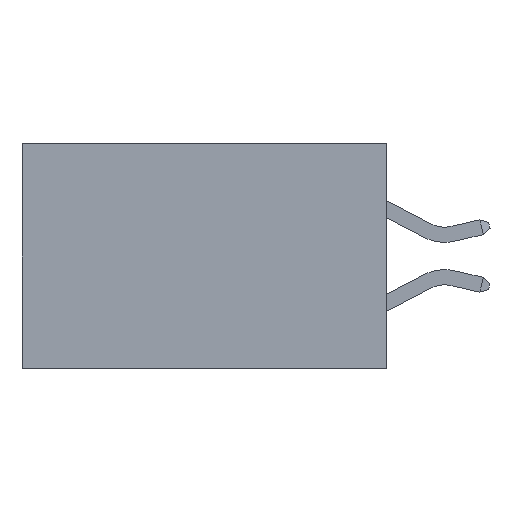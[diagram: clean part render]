
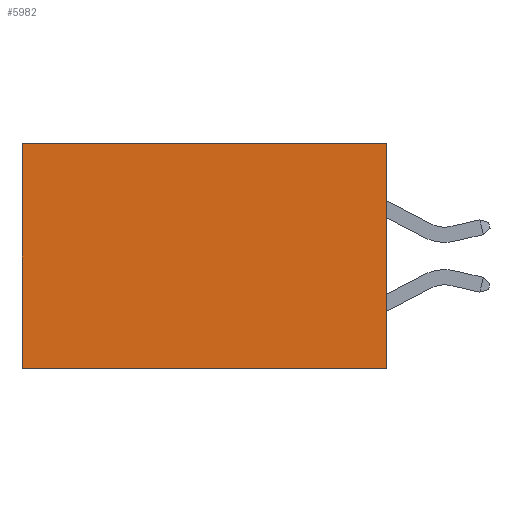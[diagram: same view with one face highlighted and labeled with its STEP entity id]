
A CAD part, left-side view. The second image highlights one B-rep face of the part: STEP entity #5982.
In plain terms, the highlighted planar face has unit normal (-1, 0, 0).
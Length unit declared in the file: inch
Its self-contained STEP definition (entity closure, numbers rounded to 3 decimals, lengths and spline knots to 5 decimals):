
#1106 = EDGE_CURVE ( 'NONE', #20716, #8782, #17215, .T. ) ;
#1130 = ORIENTED_EDGE ( 'NONE', *, *, #15446, .F. ) ;
#2892 = VERTEX_POINT ( 'NONE', #3396 ) ;
#3396 = CARTESIAN_POINT ( 'NONE',  ( 0.2615, 0., -0.37 ) ) ;
#3683 = DIRECTION ( 'NONE',  ( 0., 0., -1. ) ) ;
#3804 = PLANE ( 'NONE',  #22544 ) ;
#4416 = EDGE_CURVE ( 'NONE', #2892, #8782, #11045, .T. ) ;
#4442 = DIRECTION ( 'NONE',  ( 0., 0., -1. ) ) ;
#5888 = DIRECTION ( 'NONE',  ( 0., 0., -1. ) ) ;
#5982 = ADVANCED_FACE ( 'NONE', ( #23547 ), #3804, .F. ) ;
#6542 = VECTOR ( 'NONE', #4442, 39.37008 ) ;
#6616 = LINE ( 'NONE', #6861, #24204 ) ;
#6861 = CARTESIAN_POINT ( 'NONE',  ( 0.2615, 0., 0. ) ) ;
#7261 = VECTOR ( 'NONE', #9505, 39.37008 ) ;
#8311 = CARTESIAN_POINT ( 'NONE',  ( 0.2615, 0.6, 0. ) ) ;
#8782 = VERTEX_POINT ( 'NONE', #24409 ) ;
#9505 = DIRECTION ( 'NONE',  ( 0., 1., 0. ) ) ;
#10264 = CARTESIAN_POINT ( 'NONE',  ( 0.2615, 0., -0.37 ) ) ;
#11045 = LINE ( 'NONE', #14894, #7261 ) ;
#11678 = CARTESIAN_POINT ( 'NONE',  ( 0.2615, 0., -0.37 ) ) ;
#11791 = CARTESIAN_POINT ( 'NONE',  ( 0.2615, 0.6, -0.37 ) ) ;
#12699 = LINE ( 'NONE', #10264, #6542 ) ;
#13491 = ORIENTED_EDGE ( 'NONE', *, *, #18817, .T. ) ;
#14714 = DIRECTION ( 'NONE',  ( 0., 1., 0. ) ) ;
#14894 = CARTESIAN_POINT ( 'NONE',  ( 0.2615, 0., -0.37 ) ) ;
#14954 = CARTESIAN_POINT ( 'NONE',  ( 0.2615, 0., 0. ) ) ;
#15446 = EDGE_CURVE ( 'NONE', #17656, #2892, #12699, .T. ) ;
#15621 = EDGE_LOOP ( 'NONE', ( #19793, #23747, #1130, #13491 ) ) ;
#17215 = LINE ( 'NONE', #11791, #21458 ) ;
#17656 = VERTEX_POINT ( 'NONE', #14954 ) ;
#17830 = DIRECTION ( 'NONE',  ( 1., 0., 0. ) ) ;
#18817 = EDGE_CURVE ( 'NONE', #17656, #20716, #6616, .T. ) ;
#19793 = ORIENTED_EDGE ( 'NONE', *, *, #1106, .T. ) ;
#20716 = VERTEX_POINT ( 'NONE', #8311 ) ;
#21458 = VECTOR ( 'NONE', #3683, 39.37008 ) ;
#22544 = AXIS2_PLACEMENT_3D ( 'NONE', #11678, #17830, #5888 ) ;
#23547 = FACE_OUTER_BOUND ( 'NONE', #15621, .T. ) ;
#23747 = ORIENTED_EDGE ( 'NONE', *, *, #4416, .F. ) ;
#24204 = VECTOR ( 'NONE', #14714, 39.37008 ) ;
#24409 = CARTESIAN_POINT ( 'NONE',  ( 0.2615, 0.6, -0.37 ) ) ;
